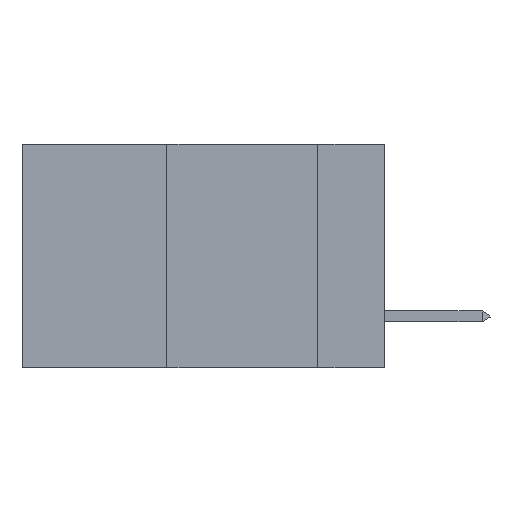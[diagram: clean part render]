
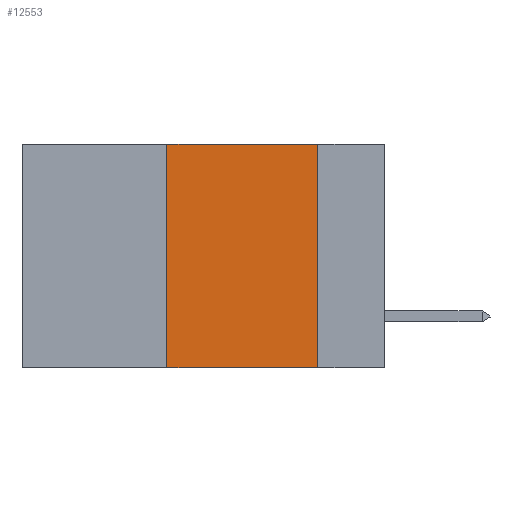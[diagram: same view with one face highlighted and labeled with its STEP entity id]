
A CAD part, left-side view. The second image highlights one B-rep face of the part: STEP entity #12553.
In plain terms, the highlighted planar face has unit normal (-1, 0, 0).
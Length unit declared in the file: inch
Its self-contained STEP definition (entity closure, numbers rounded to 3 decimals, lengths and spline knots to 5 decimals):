
#264 = DIRECTION ( 'NONE',  ( 0., 0., -1. ) ) ;
#1061 = CARTESIAN_POINT ( 'NONE',  ( 0., 0.11, -0.37 ) ) ;
#1739 = EDGE_LOOP ( 'NONE', ( #14586, #19936, #7743, #10680 ) ) ;
#2558 = CARTESIAN_POINT ( 'NONE',  ( 0., 0.6, -0.37 ) ) ;
#4641 = DIRECTION ( 'NONE',  ( 0., 0., 1. ) ) ;
#4865 = VECTOR ( 'NONE', #18804, 39.37008 ) ;
#5068 = LINE ( 'NONE', #8931, #7354 ) ;
#5327 = VERTEX_POINT ( 'NONE', #1061 ) ;
#6111 = CARTESIAN_POINT ( 'NONE',  ( 0., 0.36, -0.37 ) ) ;
#7354 = VECTOR ( 'NONE', #264, 39.37008 ) ;
#7743 = ORIENTED_EDGE ( 'NONE', *, *, #8688, .F. ) ;
#8688 = EDGE_CURVE ( 'NONE', #13954, #14959, #18365, .T. ) ;
#8931 = CARTESIAN_POINT ( 'NONE',  ( 0., 0.11, 0. ) ) ;
#9101 = DIRECTION ( 'NONE',  ( 1., 0., 0. ) ) ;
#9566 = LINE ( 'NONE', #16079, #18807 ) ;
#9664 = EDGE_CURVE ( 'NONE', #19979, #5327, #5068, .T. ) ;
#10680 = ORIENTED_EDGE ( 'NONE', *, *, #21407, .T. ) ;
#11572 = FACE_OUTER_BOUND ( 'NONE', #1739, .T. ) ;
#11871 = CARTESIAN_POINT ( 'NONE',  ( 0., 0.36, 0. ) ) ;
#12553 = ADVANCED_FACE ( 'NONE', ( #11572 ), #17930, .F. ) ;
#13954 = VERTEX_POINT ( 'NONE', #6111 ) ;
#14586 = ORIENTED_EDGE ( 'NONE', *, *, #9664, .F. ) ;
#14655 = LINE ( 'NONE', #2558, #4865 ) ;
#14680 = DIRECTION ( 'NONE',  ( 0., 0., -1. ) ) ;
#14959 = VERTEX_POINT ( 'NONE', #23384 ) ;
#16079 = CARTESIAN_POINT ( 'NONE',  ( 0., 0.6, 0. ) ) ;
#17930 = PLANE ( 'NONE',  #22044 ) ;
#18018 = DIRECTION ( 'NONE',  ( 0., -1., 0. ) ) ;
#18110 = EDGE_CURVE ( 'NONE', #14959, #19979, #9566, .T. ) ;
#18365 = LINE ( 'NONE', #11871, #22617 ) ;
#18804 = DIRECTION ( 'NONE',  ( 0., -1., 0. ) ) ;
#18807 = VECTOR ( 'NONE', #18018, 39.37008 ) ;
#19454 = CARTESIAN_POINT ( 'NONE',  ( 0., 0.11, 0. ) ) ;
#19936 = ORIENTED_EDGE ( 'NONE', *, *, #18110, .F. ) ;
#19979 = VERTEX_POINT ( 'NONE', #19454 ) ;
#21407 = EDGE_CURVE ( 'NONE', #13954, #5327, #14655, .T. ) ;
#21609 = CARTESIAN_POINT ( 'NONE',  ( 0., 0.6, 0. ) ) ;
#22044 = AXIS2_PLACEMENT_3D ( 'NONE', #21609, #9101, #14680 ) ;
#22617 = VECTOR ( 'NONE', #4641, 39.37008 ) ;
#23384 = CARTESIAN_POINT ( 'NONE',  ( 0., 0.36, 0. ) ) ;
